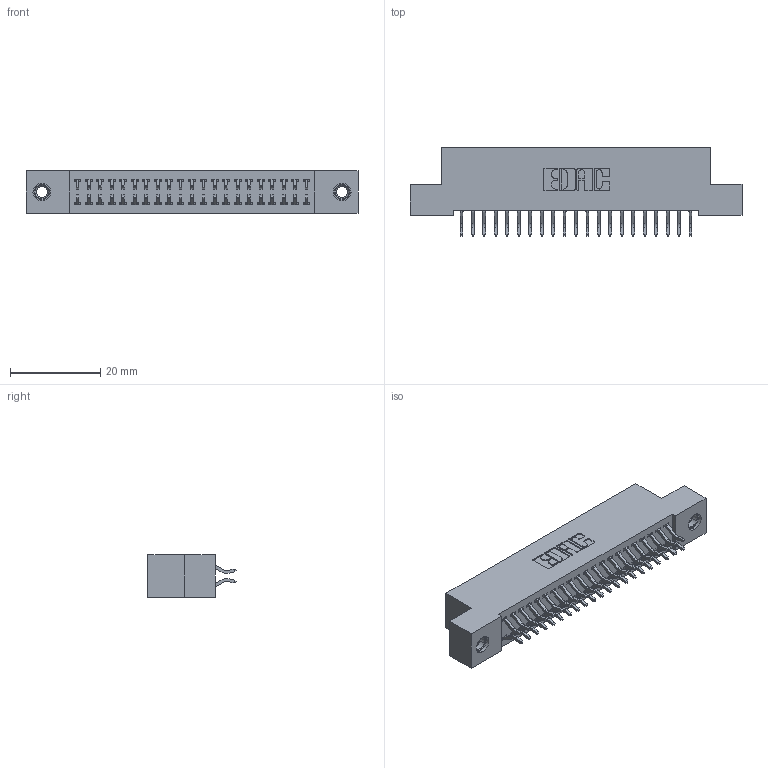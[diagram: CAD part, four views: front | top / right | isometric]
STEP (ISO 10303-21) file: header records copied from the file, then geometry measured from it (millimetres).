
FILE_DESCRIPTION (( 'STEP AP203' ), '1' );
FILE_NAME ('342-042-556-207.STEP', '2018-08-12T13:21:55', ( '' ), ( '' ), 'SwSTEP 2.0', 'SolidWorks 2016', '' );
FILE_SCHEMA (( 'CONFIG_CONTROL_DESIGN' ));
Length unit declared in the file: inch
Products named in the file (4): 342 Part_TI; 345-292-001_556 Tail; 342-042-556-207; 345-250-001_345-250-005-103
Assembly tree (45 placements, depth 2):
  342-042-556-207
    342 Part_TI
    345-292-001_556 Tail  x42
    345-250-001_345-250-005-103  x2
Bounding box: 73.66 x 19.58 x 9.4 mm (x, y, z)
Volume: 6505.2 mm3; surface area: 10056.4 mm2
Topology: 45 solids, 45 shells, 2606 faces, 7701 edges, 5070 vertices
Faces by surface type: plane 1778, cylinder 812, cone 12, torus 4
Entity records: 17500 total; most frequent: CARTESIAN_POINT 2921, ORIENTED_EDGE 2838, DIRECTION 2553, EDGE_CURVE 1419, VECTOR 1263, LINE 1263, VERTEX_POINT 940, AXIS2_PLACEMENT_3D 645
